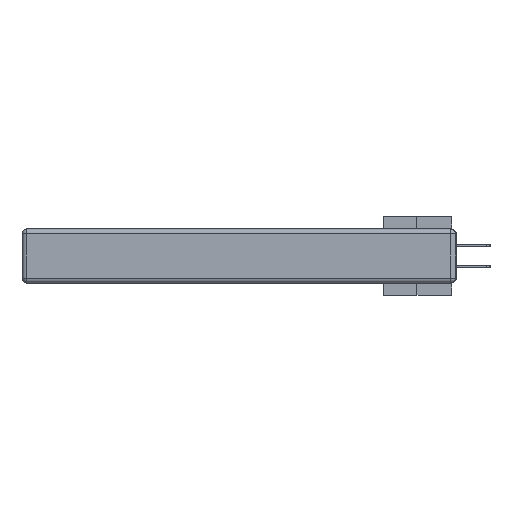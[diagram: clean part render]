
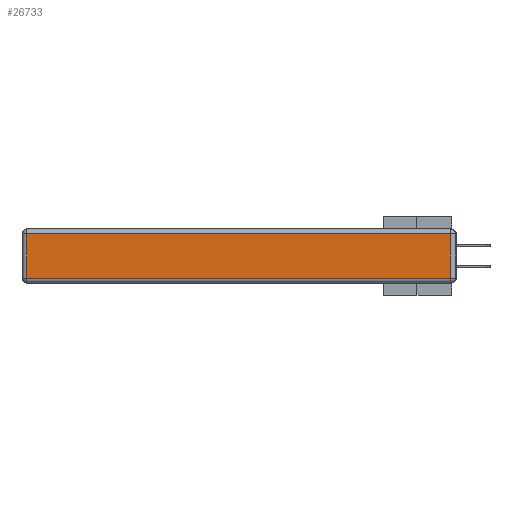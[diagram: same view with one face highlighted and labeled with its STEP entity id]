
A CAD part, left-side view. The second image highlights one B-rep face of the part: STEP entity #26733.
In plain terms, the highlighted planar face has unit normal (-1, 0, 0).
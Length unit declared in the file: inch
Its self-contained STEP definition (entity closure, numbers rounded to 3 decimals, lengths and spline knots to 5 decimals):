
#72 = LINE ( 'NONE', #24146, #16387 ) ;
#2755 = VERTEX_POINT ( 'NONE', #5667 ) ;
#5245 = EDGE_CURVE ( 'NONE', #20492, #2755, #36770, .T. ) ;
#5667 = CARTESIAN_POINT ( 'NONE',  ( 0., 0.03, -0.03 ) ) ;
#8024 = VECTOR ( 'NONE', #36975, 39.37008 ) ;
#9086 = ORIENTED_EDGE ( 'NONE', *, *, #13085, .T. ) ;
#9137 = CARTESIAN_POINT ( 'NONE',  ( 0., 0., -0.343 ) ) ;
#9455 = LINE ( 'NONE', #28023, #8024 ) ;
#12346 = DIRECTION ( 'NONE',  ( -1., 0., 0. ) ) ;
#12546 = ORIENTED_EDGE ( 'NONE', *, *, #24465, .T. ) ;
#12626 = DIRECTION ( 'NONE',  ( 0., 0., -1. ) ) ;
#13085 = EDGE_CURVE ( 'NONE', #30184, #31290, #27966, .T. ) ;
#13217 = DIRECTION ( 'NONE',  ( 0., -1., 0. ) ) ;
#14790 = EDGE_LOOP ( 'NONE', ( #12546, #32231, #33045, #9086 ) ) ;
#16387 = VECTOR ( 'NONE', #13217, 39.37008 ) ;
#18189 = DIRECTION ( 'NONE',  ( 0., 0., 1. ) ) ;
#18734 = CARTESIAN_POINT ( 'NONE',  ( 0., 2.72, -0.343 ) ) ;
#18824 = DIRECTION ( 'NONE',  ( 0., 0., 1. ) ) ;
#20032 = VECTOR ( 'NONE', #12626, 39.37008 ) ;
#20492 = VERTEX_POINT ( 'NONE', #28847 ) ;
#20656 = PLANE ( 'NONE',  #31543 ) ;
#22399 = VECTOR ( 'NONE', #18824, 39.37008 ) ;
#23450 = FACE_OUTER_BOUND ( 'NONE', #14790, .T. ) ;
#24030 = CARTESIAN_POINT ( 'NONE',  ( 0., 2.72, -0.03 ) ) ;
#24146 = CARTESIAN_POINT ( 'NONE',  ( 0., 0., -0.313 ) ) ;
#24454 = EDGE_CURVE ( 'NONE', #2755, #30184, #9455, .T. ) ;
#24465 = EDGE_CURVE ( 'NONE', #31290, #20492, #72, .T. ) ;
#26733 = ADVANCED_FACE ( 'NONE', ( #23450 ), #20656, .T. ) ;
#27966 = LINE ( 'NONE', #18734, #20032 ) ;
#28023 = CARTESIAN_POINT ( 'NONE',  ( 0., 2.75, -0.03 ) ) ;
#28847 = CARTESIAN_POINT ( 'NONE',  ( 0., 0.03, -0.313 ) ) ;
#30184 = VERTEX_POINT ( 'NONE', #24030 ) ;
#31290 = VERTEX_POINT ( 'NONE', #33407 ) ;
#31543 = AXIS2_PLACEMENT_3D ( 'NONE', #9137, #12346, #18189 ) ;
#32231 = ORIENTED_EDGE ( 'NONE', *, *, #5245, .T. ) ;
#33045 = ORIENTED_EDGE ( 'NONE', *, *, #24454, .T. ) ;
#33407 = CARTESIAN_POINT ( 'NONE',  ( 0., 2.72, -0.313 ) ) ;
#33600 = CARTESIAN_POINT ( 'NONE',  ( 0., 0.03, -0.343 ) ) ;
#36770 = LINE ( 'NONE', #33600, #22399 ) ;
#36975 = DIRECTION ( 'NONE',  ( 0., 1., 0. ) ) ;
